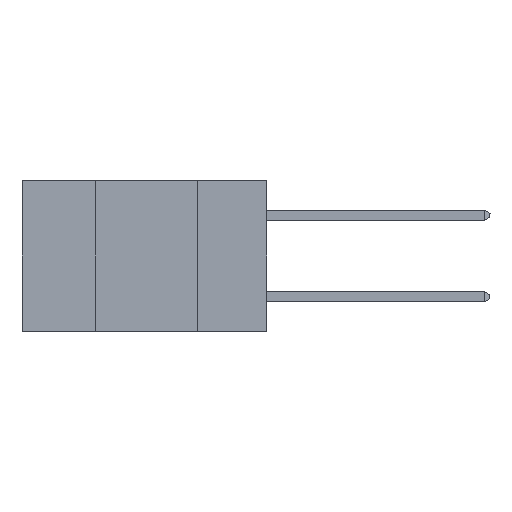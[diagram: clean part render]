
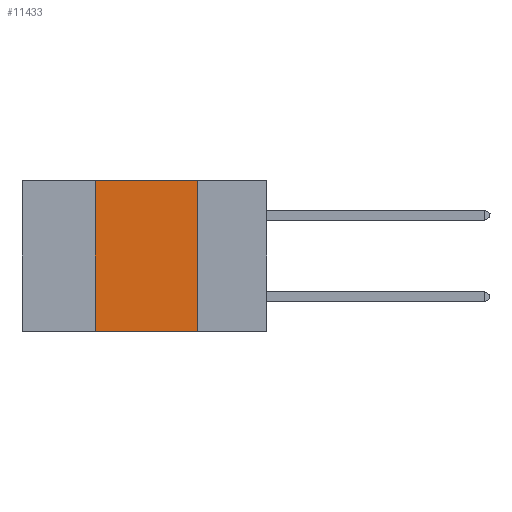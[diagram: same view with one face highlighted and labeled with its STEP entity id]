
A CAD part, left-side view. The second image highlights one B-rep face of the part: STEP entity #11433.
In plain terms, the highlighted planar face has unit normal (-1, 0, 0).
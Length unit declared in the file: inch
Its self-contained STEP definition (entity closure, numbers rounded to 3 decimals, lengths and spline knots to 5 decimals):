
#427 = ORIENTED_EDGE ( 'NONE', *, *, #7084, .T. ) ;
#562 = CARTESIAN_POINT ( 'NONE',  ( 0., 0.42, -0.37 ) ) ;
#832 = DIRECTION ( 'NONE',  ( 0., -1., 0. ) ) ;
#839 = CARTESIAN_POINT ( 'NONE',  ( 0., 0.42, 0. ) ) ;
#992 = VECTOR ( 'NONE', #5997, 39.37008 ) ;
#1025 = EDGE_CURVE ( 'NONE', #7489, #6023, #8747, .T. ) ;
#1148 = ORIENTED_EDGE ( 'NONE', *, *, #1025, .F. ) ;
#1415 = ORIENTED_EDGE ( 'NONE', *, *, #3789, .F. ) ;
#1590 = DIRECTION ( 'NONE',  ( 0., -1., 0. ) ) ;
#1810 = PLANE ( 'NONE',  #10874 ) ;
#3692 = EDGE_LOOP ( 'NONE', ( #1148, #6300, #1415, #427 ) ) ;
#3789 = EDGE_CURVE ( 'NONE', #5180, #6615, #11422, .T. ) ;
#5180 = VERTEX_POINT ( 'NONE', #562 ) ;
#5555 = CARTESIAN_POINT ( 'NONE',  ( 0., 0.17, 0. ) ) ;
#5997 = DIRECTION ( 'NONE',  ( 0., 0., 1. ) ) ;
#6012 = LINE ( 'NONE', #11096, #10990 ) ;
#6023 = VERTEX_POINT ( 'NONE', #10139 ) ;
#6300 = ORIENTED_EDGE ( 'NONE', *, *, #9435, .F. ) ;
#6615 = VERTEX_POINT ( 'NONE', #839 ) ;
#6681 = LINE ( 'NONE', #8034, #7986 ) ;
#7084 = EDGE_CURVE ( 'NONE', #5180, #6023, #6681, .T. ) ;
#7479 = DIRECTION ( 'NONE',  ( 0., 0., -1. ) ) ;
#7489 = VERTEX_POINT ( 'NONE', #5555 ) ;
#7986 = VECTOR ( 'NONE', #1590, 39.37008 ) ;
#8034 = CARTESIAN_POINT ( 'NONE',  ( 0., 0.6, -0.37 ) ) ;
#8364 = DIRECTION ( 'NONE',  ( 1., 0., 0. ) ) ;
#8747 = LINE ( 'NONE', #12181, #12001 ) ;
#9395 = DIRECTION ( 'NONE',  ( 0., 0., -1. ) ) ;
#9435 = EDGE_CURVE ( 'NONE', #6615, #7489, #6012, .T. ) ;
#10139 = CARTESIAN_POINT ( 'NONE',  ( 0., 0.17, -0.37 ) ) ;
#10220 = FACE_OUTER_BOUND ( 'NONE', #3692, .T. ) ;
#10609 = CARTESIAN_POINT ( 'NONE',  ( 0., 0.42, 0. ) ) ;
#10874 = AXIS2_PLACEMENT_3D ( 'NONE', #12156, #8364, #9395 ) ;
#10990 = VECTOR ( 'NONE', #832, 39.37008 ) ;
#11096 = CARTESIAN_POINT ( 'NONE',  ( 0., 0.6, 0. ) ) ;
#11422 = LINE ( 'NONE', #10609, #992 ) ;
#11433 = ADVANCED_FACE ( 'NONE', ( #10220 ), #1810, .F. ) ;
#12001 = VECTOR ( 'NONE', #7479, 39.37008 ) ;
#12156 = CARTESIAN_POINT ( 'NONE',  ( 0., 0.6, 0. ) ) ;
#12181 = CARTESIAN_POINT ( 'NONE',  ( 0., 0.17, 0. ) ) ;
